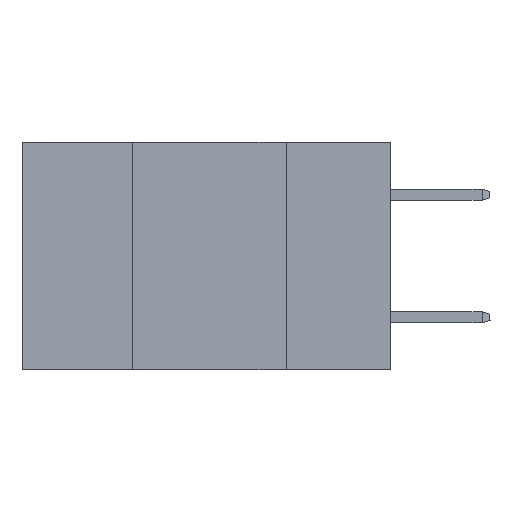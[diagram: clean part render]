
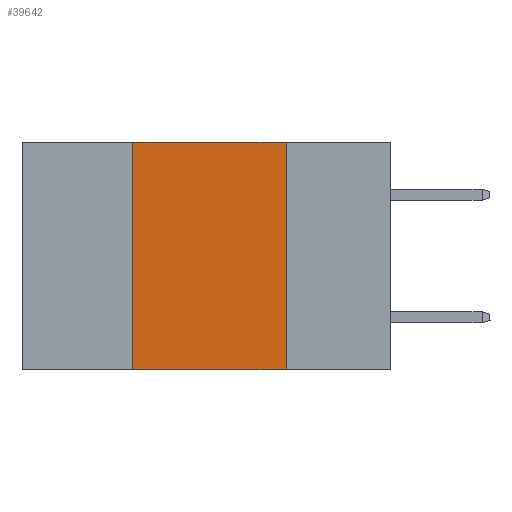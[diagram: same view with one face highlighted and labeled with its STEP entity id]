
A CAD part, left-side view. The second image highlights one B-rep face of the part: STEP entity #39642.
In plain terms, the highlighted planar face has unit normal (-1, 0, 0).
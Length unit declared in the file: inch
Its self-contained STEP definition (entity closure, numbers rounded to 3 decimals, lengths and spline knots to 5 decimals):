
#630 = LINE ( 'NONE', #9197, #21071 ) ;
#749 = EDGE_CURVE ( 'NONE', #37171, #37685, #8994, .T. ) ;
#3242 = VECTOR ( 'NONE', #18997, 39.37008 ) ;
#3820 = CARTESIAN_POINT ( 'NONE',  ( 0., 0.6, 0. ) ) ;
#4663 = ORIENTED_EDGE ( 'NONE', *, *, #20060, .T. ) ;
#5686 = CARTESIAN_POINT ( 'NONE',  ( 0., 0.17, 0. ) ) ;
#6290 = LINE ( 'NONE', #14262, #24655 ) ;
#6824 = PLANE ( 'NONE',  #7161 ) ;
#7161 = AXIS2_PLACEMENT_3D ( 'NONE', #3820, #39603, #19632 ) ;
#7296 = ORIENTED_EDGE ( 'NONE', *, *, #24760, .F. ) ;
#7401 = FACE_OUTER_BOUND ( 'NONE', #39542, .T. ) ;
#8994 = LINE ( 'NONE', #40239, #9483 ) ;
#9197 = CARTESIAN_POINT ( 'NONE',  ( 0., 0.17, 0. ) ) ;
#9483 = VECTOR ( 'NONE', #20712, 39.37008 ) ;
#10182 = EDGE_CURVE ( 'NONE', #37685, #30764, #630, .T. ) ;
#13027 = DIRECTION ( 'NONE',  ( 0., 0., -1. ) ) ;
#14262 = CARTESIAN_POINT ( 'NONE',  ( 0., 0.6, -0.37 ) ) ;
#15050 = VERTEX_POINT ( 'NONE', #24177 ) ;
#16270 = ORIENTED_EDGE ( 'NONE', *, *, #10182, .F. ) ;
#17829 = ORIENTED_EDGE ( 'NONE', *, *, #749, .F. ) ;
#18997 = DIRECTION ( 'NONE',  ( 0., 0., 1. ) ) ;
#19632 = DIRECTION ( 'NONE',  ( 0., 0., -1. ) ) ;
#20060 = EDGE_CURVE ( 'NONE', #15050, #30764, #6290, .T. ) ;
#20712 = DIRECTION ( 'NONE',  ( 0., -1., 0. ) ) ;
#21071 = VECTOR ( 'NONE', #13027, 39.37008 ) ;
#22294 = CARTESIAN_POINT ( 'NONE',  ( 0., 0.42, 0. ) ) ;
#24177 = CARTESIAN_POINT ( 'NONE',  ( 0., 0.42, -0.37 ) ) ;
#24655 = VECTOR ( 'NONE', #41414, 39.37008 ) ;
#24760 = EDGE_CURVE ( 'NONE', #15050, #37171, #28245, .T. ) ;
#28245 = LINE ( 'NONE', #22294, #3242 ) ;
#29813 = CARTESIAN_POINT ( 'NONE',  ( 0., 0.42, 0. ) ) ;
#30362 = CARTESIAN_POINT ( 'NONE',  ( 0., 0.17, -0.37 ) ) ;
#30764 = VERTEX_POINT ( 'NONE', #30362 ) ;
#37171 = VERTEX_POINT ( 'NONE', #29813 ) ;
#37685 = VERTEX_POINT ( 'NONE', #5686 ) ;
#39542 = EDGE_LOOP ( 'NONE', ( #16270, #17829, #7296, #4663 ) ) ;
#39603 = DIRECTION ( 'NONE',  ( 1., 0., 0. ) ) ;
#39642 = ADVANCED_FACE ( 'NONE', ( #7401 ), #6824, .F. ) ;
#40239 = CARTESIAN_POINT ( 'NONE',  ( 0., 0.6, 0. ) ) ;
#41414 = DIRECTION ( 'NONE',  ( 0., -1., 0. ) ) ;
